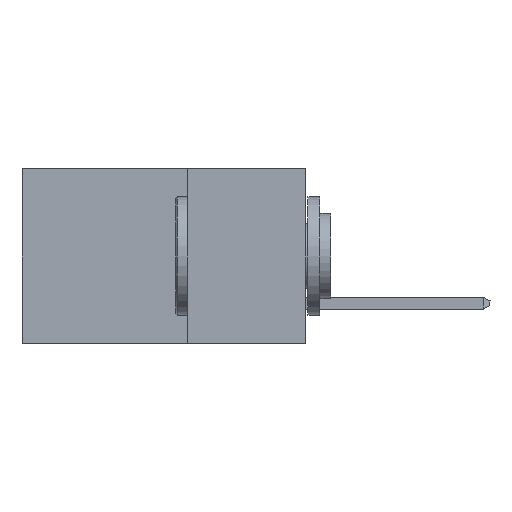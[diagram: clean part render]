
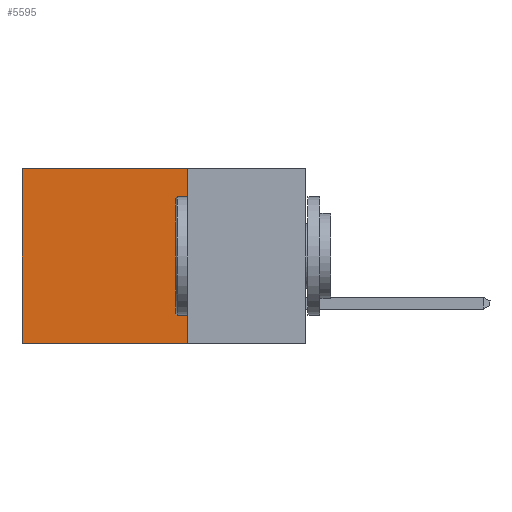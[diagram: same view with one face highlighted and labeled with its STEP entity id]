
A CAD part, left-side view. The second image highlights one B-rep face of the part: STEP entity #5595.
In plain terms, the highlighted planar face has unit normal (-1, 0, 0).
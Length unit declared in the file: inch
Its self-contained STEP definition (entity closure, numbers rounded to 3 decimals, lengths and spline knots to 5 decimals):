
#121 = EDGE_CURVE ( 'NONE', #12442, #2975, #16995, .T. ) ;
#738 = LINE ( 'NONE', #14142, #12436 ) ;
#2191 = EDGE_CURVE ( 'NONE', #15954, #12442, #16236, .T. ) ;
#2664 = PLANE ( 'NONE',  #3231 ) ;
#2750 = DIRECTION ( 'NONE',  ( 1., 0., 0. ) ) ;
#2975 = VERTEX_POINT ( 'NONE', #9460 ) ;
#3231 = AXIS2_PLACEMENT_3D ( 'NONE', #5564, #2750, #13385 ) ;
#4206 = DIRECTION ( 'NONE',  ( 0., 1., 0. ) ) ;
#4929 = VECTOR ( 'NONE', #4206, 39.37008 ) ;
#5105 = DIRECTION ( 'NONE',  ( 0., 1., 0. ) ) ;
#5564 = CARTESIAN_POINT ( 'NONE',  ( 0.2615, 0.25, -0.37 ) ) ;
#5595 = ADVANCED_FACE ( 'NONE', ( #12619 ), #2664, .F. ) ;
#5955 = ORIENTED_EDGE ( 'NONE', *, *, #121, .T. ) ;
#6312 = EDGE_LOOP ( 'NONE', ( #5955, #8879, #14317, #14238 ) ) ;
#6322 = EDGE_CURVE ( 'NONE', #16772, #2975, #738, .T. ) ;
#6425 = CARTESIAN_POINT ( 'NONE',  ( 0.2615, 0.25, 0. ) ) ;
#7783 = CARTESIAN_POINT ( 'NONE',  ( 0.2615, 0.6, 0. ) ) ;
#7818 = CARTESIAN_POINT ( 'NONE',  ( 0.2615, 0.25, -0.37 ) ) ;
#8690 = DIRECTION ( 'NONE',  ( 0., 0., -1. ) ) ;
#8879 = ORIENTED_EDGE ( 'NONE', *, *, #6322, .F. ) ;
#9460 = CARTESIAN_POINT ( 'NONE',  ( 0.2615, 0.6, -0.37 ) ) ;
#9812 = VECTOR ( 'NONE', #8690, 39.37008 ) ;
#10641 = CARTESIAN_POINT ( 'NONE',  ( 0.2615, 0.6, -0.37 ) ) ;
#12436 = VECTOR ( 'NONE', #5105, 39.37008 ) ;
#12442 = VERTEX_POINT ( 'NONE', #7783 ) ;
#12619 = FACE_OUTER_BOUND ( 'NONE', #6312, .T. ) ;
#12677 = CARTESIAN_POINT ( 'NONE',  ( 0.2615, 0.25, -0.37 ) ) ;
#13385 = DIRECTION ( 'NONE',  ( 0., 0., -1. ) ) ;
#13884 = VECTOR ( 'NONE', #16023, 39.37008 ) ;
#14119 = CARTESIAN_POINT ( 'NONE',  ( 0.2615, 0.25, 0. ) ) ;
#14142 = CARTESIAN_POINT ( 'NONE',  ( 0.2615, 0.25, -0.37 ) ) ;
#14238 = ORIENTED_EDGE ( 'NONE', *, *, #2191, .T. ) ;
#14317 = ORIENTED_EDGE ( 'NONE', *, *, #14748, .F. ) ;
#14748 = EDGE_CURVE ( 'NONE', #15954, #16772, #15366, .T. ) ;
#15366 = LINE ( 'NONE', #12677, #9812 ) ;
#15954 = VERTEX_POINT ( 'NONE', #14119 ) ;
#16023 = DIRECTION ( 'NONE',  ( 0., 0., -1. ) ) ;
#16236 = LINE ( 'NONE', #6425, #4929 ) ;
#16772 = VERTEX_POINT ( 'NONE', #7818 ) ;
#16995 = LINE ( 'NONE', #10641, #13884 ) ;
